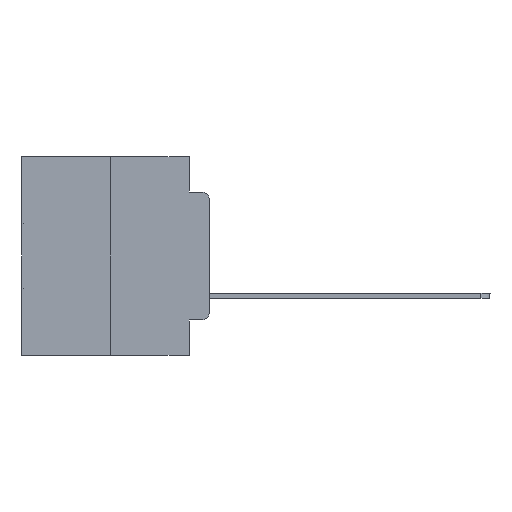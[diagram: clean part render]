
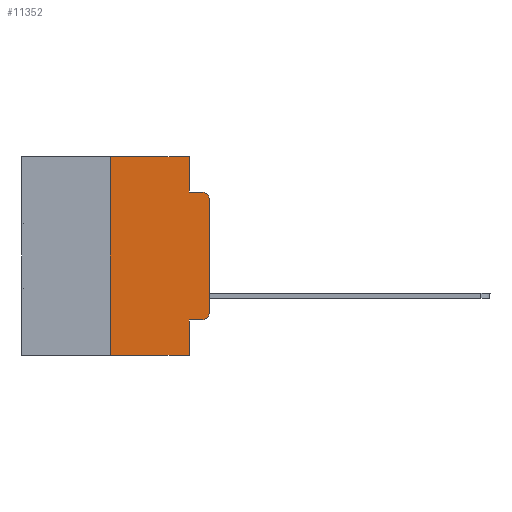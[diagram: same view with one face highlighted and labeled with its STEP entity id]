
A CAD part, left-side view. The second image highlights one B-rep face of the part: STEP entity #11352.
In plain terms, the highlighted planar face has unit normal (-1, 0, 0).
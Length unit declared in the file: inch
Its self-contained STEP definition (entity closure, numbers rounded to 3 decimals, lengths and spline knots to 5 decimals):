
#278 = CARTESIAN_POINT ( 'NONE',  ( 0., 0.25, -0.5 ) ) ;
#309 = DIRECTION ( 'NONE',  ( 0., 0., 1. ) ) ;
#488 = CARTESIAN_POINT ( 'NONE',  ( 0., 0.051, -0.4115 ) ) ;
#1087 = ORIENTED_EDGE ( 'NONE', *, *, #13313, .F. ) ;
#1809 = EDGE_CURVE ( 'NONE', #8869, #20769, #29396, .T. ) ;
#2027 = EDGE_CURVE ( 'NONE', #2890, #25371, #10869, .T. ) ;
#2087 = CARTESIAN_POINT ( 'NONE',  ( 0., 0.02, -0.3915 ) ) ;
#2196 = DIRECTION ( 'NONE',  ( -1., 0., 0. ) ) ;
#2381 = VERTEX_POINT ( 'NONE', #15520 ) ;
#2420 = CARTESIAN_POINT ( 'NONE',  ( 0., 0.25, 0. ) ) ;
#2805 = CARTESIAN_POINT ( 'NONE',  ( 0., 0.25, 0. ) ) ;
#2890 = VERTEX_POINT ( 'NONE', #2805 ) ;
#2938 = VECTOR ( 'NONE', #10202, 39.37008 ) ;
#3647 = CARTESIAN_POINT ( 'NONE',  ( 0., 0.473, 0. ) ) ;
#3972 = DIRECTION ( 'NONE',  ( 0., -1., 0. ) ) ;
#4257 = EDGE_CURVE ( 'NONE', #31276, #14263, #21738, .T. ) ;
#4379 = CARTESIAN_POINT ( 'NONE',  ( 0., 0.051, -0.4115 ) ) ;
#4443 = VECTOR ( 'NONE', #3972, 39.37008 ) ;
#5527 = VECTOR ( 'NONE', #29238, 39.37008 ) ;
#5548 = CARTESIAN_POINT ( 'NONE',  ( 0., 0., -0.3915 ) ) ;
#5555 = DIRECTION ( 'NONE',  ( 0., 0., -1. ) ) ;
#6181 = DIRECTION ( 'NONE',  ( 0., -1., 0. ) ) ;
#6386 = CIRCLE ( 'NONE', #22424, 0.02 ) ;
#6457 = CARTESIAN_POINT ( 'NONE',  ( 0., 0.02, -0.4115 ) ) ;
#6767 = CARTESIAN_POINT ( 'NONE',  ( 0., 0.02, -0.0885 ) ) ;
#7325 = DIRECTION ( 'NONE',  ( 1., 0., 0. ) ) ;
#7470 = CARTESIAN_POINT ( 'NONE',  ( 0., 0., 0. ) ) ;
#8161 = LINE ( 'NONE', #13272, #10029 ) ;
#8869 = VERTEX_POINT ( 'NONE', #5548 ) ;
#9408 = EDGE_CURVE ( 'NONE', #2381, #22440, #23274, .T. ) ;
#9490 = EDGE_CURVE ( 'NONE', #27929, #2890, #30078, .T. ) ;
#9916 = DIRECTION ( 'NONE',  ( -1., 0., 0. ) ) ;
#10029 = VECTOR ( 'NONE', #6181, 39.37008 ) ;
#10202 = DIRECTION ( 'NONE',  ( 0., 0., 1. ) ) ;
#10869 = LINE ( 'NONE', #3647, #4443 ) ;
#10886 = VECTOR ( 'NONE', #5555, 39.37008 ) ;
#11352 = ADVANCED_FACE ( 'NONE', ( #19049 ), #28764, .F. ) ;
#11791 = CARTESIAN_POINT ( 'NONE',  ( 0., 0.051, -0.5 ) ) ;
#11804 = ORIENTED_EDGE ( 'NONE', *, *, #9408, .F. ) ;
#12327 = EDGE_CURVE ( 'NONE', #14263, #8869, #17850, .T. ) ;
#12622 = EDGE_CURVE ( 'NONE', #25371, #2381, #22615, .T. ) ;
#13272 = CARTESIAN_POINT ( 'NONE',  ( 0., 0.473, -0.5 ) ) ;
#13313 = EDGE_CURVE ( 'NONE', #31276, #30933, #17660, .T. ) ;
#14263 = VERTEX_POINT ( 'NONE', #6457 ) ;
#14931 = EDGE_LOOP ( 'NONE', ( #19690, #17749, #11804, #18350, #22384, #25605, #20614, #1087, #23148, #15802 ) ) ;
#15312 = VECTOR ( 'NONE', #21547, 39.37008 ) ;
#15520 = CARTESIAN_POINT ( 'NONE',  ( 0., 0.051, -0.0885 ) ) ;
#15802 = ORIENTED_EDGE ( 'NONE', *, *, #12327, .T. ) ;
#16810 = AXIS2_PLACEMENT_3D ( 'NONE', #24117, #7325, #28867 ) ;
#17516 = CARTESIAN_POINT ( 'NONE',  ( 0., 0.051, 0. ) ) ;
#17660 = LINE ( 'NONE', #19547, #5527 ) ;
#17747 = CARTESIAN_POINT ( 'NONE',  ( 0., 0.051, -0.0885 ) ) ;
#17749 = ORIENTED_EDGE ( 'NONE', *, *, #30588, .T. ) ;
#17850 = CIRCLE ( 'NONE', #26745, 0.02 ) ;
#18350 = ORIENTED_EDGE ( 'NONE', *, *, #12622, .F. ) ;
#19049 = FACE_OUTER_BOUND ( 'NONE', #14931, .T. ) ;
#19547 = CARTESIAN_POINT ( 'NONE',  ( 0., 0.051, 0. ) ) ;
#19690 = ORIENTED_EDGE ( 'NONE', *, *, #1809, .T. ) ;
#19889 = VECTOR ( 'NONE', #309, 39.37008 ) ;
#20081 = CARTESIAN_POINT ( 'NONE',  ( 0., 0.02, -0.1085 ) ) ;
#20281 = DIRECTION ( 'NONE',  ( 0., -1., 0. ) ) ;
#20614 = ORIENTED_EDGE ( 'NONE', *, *, #20845, .T. ) ;
#20769 = VERTEX_POINT ( 'NONE', #29215 ) ;
#20845 = EDGE_CURVE ( 'NONE', #27929, #30933, #8161, .T. ) ;
#21547 = DIRECTION ( 'NONE',  ( 0., -1., 0. ) ) ;
#21738 = LINE ( 'NONE', #4379, #15312 ) ;
#22384 = ORIENTED_EDGE ( 'NONE', *, *, #2027, .F. ) ;
#22424 = AXIS2_PLACEMENT_3D ( 'NONE', #20081, #9916, #27138 ) ;
#22440 = VERTEX_POINT ( 'NONE', #6767 ) ;
#22615 = LINE ( 'NONE', #17516, #10886 ) ;
#23148 = ORIENTED_EDGE ( 'NONE', *, *, #4257, .T. ) ;
#23274 = LINE ( 'NONE', #17747, #29678 ) ;
#24117 = CARTESIAN_POINT ( 'NONE',  ( 0., 0.473, 0. ) ) ;
#25371 = VERTEX_POINT ( 'NONE', #27155 ) ;
#25605 = ORIENTED_EDGE ( 'NONE', *, *, #9490, .F. ) ;
#26079 = DIRECTION ( 'NONE',  ( 0., 0., -1. ) ) ;
#26745 = AXIS2_PLACEMENT_3D ( 'NONE', #2087, #2196, #26079 ) ;
#27138 = DIRECTION ( 'NONE',  ( 0., 0., -1. ) ) ;
#27155 = CARTESIAN_POINT ( 'NONE',  ( 0., 0.051, 0. ) ) ;
#27929 = VERTEX_POINT ( 'NONE', #278 ) ;
#28764 = PLANE ( 'NONE',  #16810 ) ;
#28867 = DIRECTION ( 'NONE',  ( 0., 0., -1. ) ) ;
#29215 = CARTESIAN_POINT ( 'NONE',  ( 0., 0., -0.1085 ) ) ;
#29238 = DIRECTION ( 'NONE',  ( 0., 0., -1. ) ) ;
#29396 = LINE ( 'NONE', #7470, #2938 ) ;
#29678 = VECTOR ( 'NONE', #20281, 39.37008 ) ;
#30078 = LINE ( 'NONE', #2420, #19889 ) ;
#30588 = EDGE_CURVE ( 'NONE', #20769, #22440, #6386, .T. ) ;
#30933 = VERTEX_POINT ( 'NONE', #11791 ) ;
#31276 = VERTEX_POINT ( 'NONE', #488 ) ;
